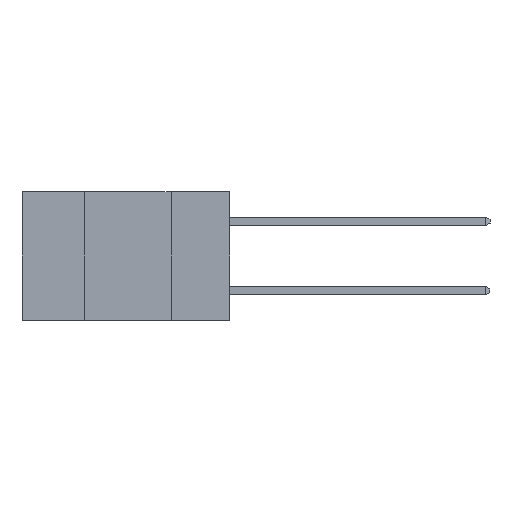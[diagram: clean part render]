
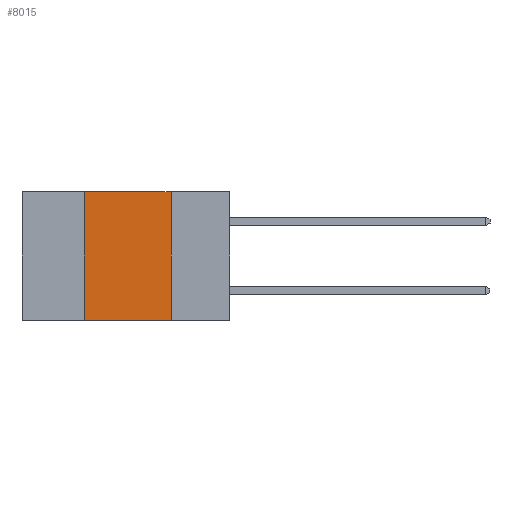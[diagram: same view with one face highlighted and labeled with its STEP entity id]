
A CAD part, left-side view. The second image highlights one B-rep face of the part: STEP entity #8015.
In plain terms, the highlighted planar face has unit normal (-1, 0, 0).
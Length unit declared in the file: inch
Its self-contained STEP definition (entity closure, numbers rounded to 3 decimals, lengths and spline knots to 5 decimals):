
#90 = LINE ( 'NONE', #8050, #12143 ) ;
#168 = DIRECTION ( 'NONE',  ( 0., 0., -1. ) ) ;
#208 = VECTOR ( 'NONE', #3478, 39.37008 ) ;
#536 = VECTOR ( 'NONE', #5598, 39.37008 ) ;
#712 = AXIS2_PLACEMENT_3D ( 'NONE', #13716, #6817, #6049 ) ;
#763 = CARTESIAN_POINT ( 'NONE',  ( 0., 0.17, -0.37 ) ) ;
#1010 = CARTESIAN_POINT ( 'NONE',  ( 0., 0.42, 0. ) ) ;
#1973 = EDGE_CURVE ( 'NONE', #4227, #3212, #13071, .T. ) ;
#3212 = VERTEX_POINT ( 'NONE', #763 ) ;
#3478 = DIRECTION ( 'NONE',  ( 0., -1., 0. ) ) ;
#3502 = LINE ( 'NONE', #1010, #536 ) ;
#4013 = VECTOR ( 'NONE', #168, 39.37008 ) ;
#4087 = CARTESIAN_POINT ( 'NONE',  ( 0., 0.42, -0.37 ) ) ;
#4227 = VERTEX_POINT ( 'NONE', #8021 ) ;
#5009 = EDGE_LOOP ( 'NONE', ( #12668, #8518, #7441, #14371 ) ) ;
#5598 = DIRECTION ( 'NONE',  ( 0., 0., 1. ) ) ;
#6049 = DIRECTION ( 'NONE',  ( 0., 0., -1. ) ) ;
#6603 = VERTEX_POINT ( 'NONE', #10853 ) ;
#6817 = DIRECTION ( 'NONE',  ( 1., 0., 0. ) ) ;
#7136 = CARTESIAN_POINT ( 'NONE',  ( 0., 0.17, 0. ) ) ;
#7441 = ORIENTED_EDGE ( 'NONE', *, *, #14311, .F. ) ;
#7549 = VERTEX_POINT ( 'NONE', #4087 ) ;
#8015 = ADVANCED_FACE ( 'NONE', ( #13050 ), #9408, .F. ) ;
#8021 = CARTESIAN_POINT ( 'NONE',  ( 0., 0.17, 0. ) ) ;
#8033 = DIRECTION ( 'NONE',  ( 0., -1., 0. ) ) ;
#8050 = CARTESIAN_POINT ( 'NONE',  ( 0., 0.6, -0.37 ) ) ;
#8518 = ORIENTED_EDGE ( 'NONE', *, *, #11854, .F. ) ;
#9255 = EDGE_CURVE ( 'NONE', #7549, #3212, #90, .T. ) ;
#9334 = LINE ( 'NONE', #12575, #208 ) ;
#9408 = PLANE ( 'NONE',  #712 ) ;
#10853 = CARTESIAN_POINT ( 'NONE',  ( 0., 0.42, 0. ) ) ;
#11854 = EDGE_CURVE ( 'NONE', #6603, #4227, #9334, .T. ) ;
#12143 = VECTOR ( 'NONE', #8033, 39.37008 ) ;
#12575 = CARTESIAN_POINT ( 'NONE',  ( 0., 0.6, 0. ) ) ;
#12668 = ORIENTED_EDGE ( 'NONE', *, *, #1973, .F. ) ;
#13050 = FACE_OUTER_BOUND ( 'NONE', #5009, .T. ) ;
#13071 = LINE ( 'NONE', #7136, #4013 ) ;
#13716 = CARTESIAN_POINT ( 'NONE',  ( 0., 0.6, 0. ) ) ;
#14311 = EDGE_CURVE ( 'NONE', #7549, #6603, #3502, .T. ) ;
#14371 = ORIENTED_EDGE ( 'NONE', *, *, #9255, .T. ) ;
